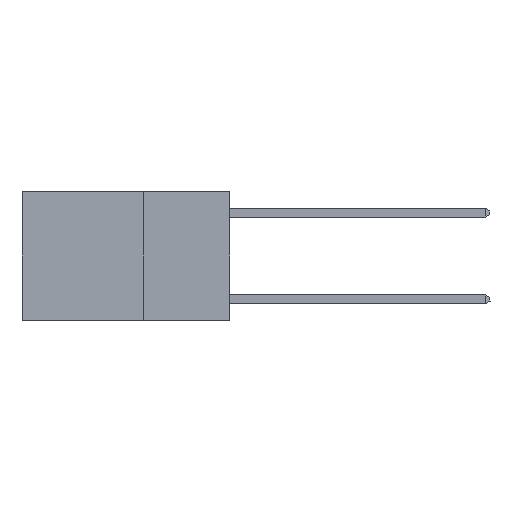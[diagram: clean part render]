
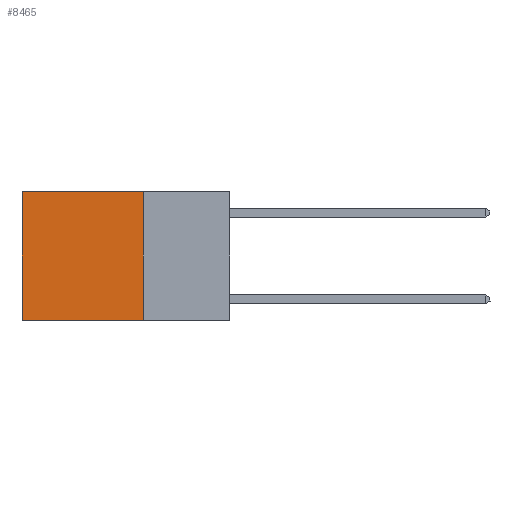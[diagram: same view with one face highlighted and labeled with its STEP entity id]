
A CAD part, left-side view. The second image highlights one B-rep face of the part: STEP entity #8465.
In plain terms, the highlighted planar face has unit normal (-1, 0, 0).
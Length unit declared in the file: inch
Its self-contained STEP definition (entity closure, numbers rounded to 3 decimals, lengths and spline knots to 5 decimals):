
#210 = CARTESIAN_POINT ( 'NONE',  ( 0.2625, 0.25, -0.37 ) ) ;
#465 = CARTESIAN_POINT ( 'NONE',  ( 0.2625, 0.25, 0. ) ) ;
#472 = CARTESIAN_POINT ( 'NONE',  ( 0.2625, 0.6, 0. ) ) ;
#2292 = DIRECTION ( 'NONE',  ( 0., 1., 0. ) ) ;
#2332 = CARTESIAN_POINT ( 'NONE',  ( 0.2625, 0.25, -0.37 ) ) ;
#2547 = ORIENTED_EDGE ( 'NONE', *, *, #4168, .T. ) ;
#3296 = EDGE_CURVE ( 'NONE', #11473, #11617, #5012, .T. ) ;
#3890 = CARTESIAN_POINT ( 'NONE',  ( 0.2625, 0.25, 0. ) ) ;
#3914 = LINE ( 'NONE', #472, #11228 ) ;
#4149 = VERTEX_POINT ( 'NONE', #16052 ) ;
#4168 = EDGE_CURVE ( 'NONE', #11617, #4149, #3914, .T. ) ;
#4821 = EDGE_CURVE ( 'NONE', #11473, #9428, #14349, .T. ) ;
#5012 = LINE ( 'NONE', #11513, #16989 ) ;
#8450 = PLANE ( 'NONE',  #11379 ) ;
#8465 = ADVANCED_FACE ( 'NONE', ( #16450 ), #8450, .F. ) ;
#8746 = EDGE_LOOP ( 'NONE', ( #2547, #10644, #15132, #10258 ) ) ;
#9428 = VERTEX_POINT ( 'NONE', #210 ) ;
#9911 = DIRECTION ( 'NONE',  ( 0., 0., -1. ) ) ;
#10012 = DIRECTION ( 'NONE',  ( 0., 0., -1. ) ) ;
#10258 = ORIENTED_EDGE ( 'NONE', *, *, #3296, .T. ) ;
#10644 = ORIENTED_EDGE ( 'NONE', *, *, #13027, .F. ) ;
#11152 = DIRECTION ( 'NONE',  ( 0., 0., -1. ) ) ;
#11228 = VECTOR ( 'NONE', #9911, 39.37008 ) ;
#11307 = LINE ( 'NONE', #2332, #12035 ) ;
#11315 = CARTESIAN_POINT ( 'NONE',  ( 0.2625, 0.25, 0. ) ) ;
#11379 = AXIS2_PLACEMENT_3D ( 'NONE', #3890, #19389, #10012 ) ;
#11473 = VERTEX_POINT ( 'NONE', #11315 ) ;
#11513 = CARTESIAN_POINT ( 'NONE',  ( 0.2625, 0.25, 0. ) ) ;
#11617 = VERTEX_POINT ( 'NONE', #15669 ) ;
#12035 = VECTOR ( 'NONE', #19410, 39.37008 ) ;
#13027 = EDGE_CURVE ( 'NONE', #9428, #4149, #11307, .T. ) ;
#14349 = LINE ( 'NONE', #465, #14612 ) ;
#14612 = VECTOR ( 'NONE', #11152, 39.37008 ) ;
#15132 = ORIENTED_EDGE ( 'NONE', *, *, #4821, .F. ) ;
#15669 = CARTESIAN_POINT ( 'NONE',  ( 0.2625, 0.6, 0. ) ) ;
#16052 = CARTESIAN_POINT ( 'NONE',  ( 0.2625, 0.6, -0.37 ) ) ;
#16450 = FACE_OUTER_BOUND ( 'NONE', #8746, .T. ) ;
#16989 = VECTOR ( 'NONE', #2292, 39.37008 ) ;
#19389 = DIRECTION ( 'NONE',  ( 1., 0., 0. ) ) ;
#19410 = DIRECTION ( 'NONE',  ( 0., 1., 0. ) ) ;
